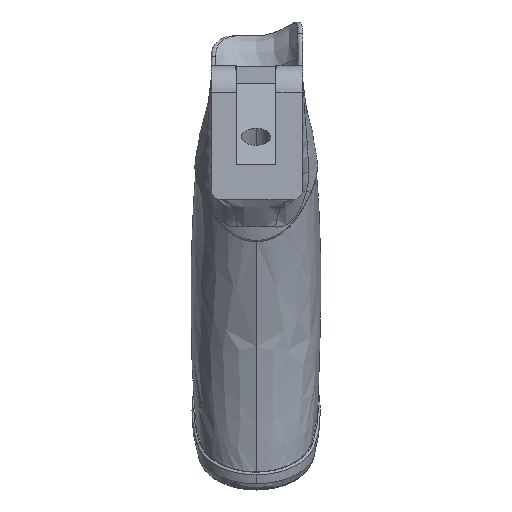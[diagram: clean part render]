
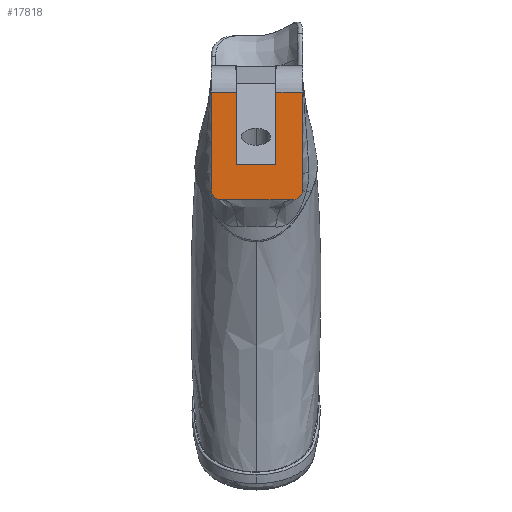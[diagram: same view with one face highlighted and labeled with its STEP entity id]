
A CAD part, top view. The second image highlights one B-rep face of the part: STEP entity #17818.
In plain terms, the highlighted planar face has unit normal (0, 0, 1).
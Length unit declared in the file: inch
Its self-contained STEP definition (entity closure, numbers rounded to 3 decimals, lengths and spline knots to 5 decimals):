
#292 = PLANE ( 'NONE',  #8919 ) ;
#348 = DIRECTION ( 'NONE',  ( 1., 0., 0. ) ) ;
#401 = CARTESIAN_POINT ( 'NONE',  ( -0.33, -1.2789, 0. ) ) ;
#866 = VERTEX_POINT ( 'NONE', #1141 ) ;
#1141 = CARTESIAN_POINT ( 'NONE',  ( 0.1875, -0.94, 0. ) ) ;
#1233 = CARTESIAN_POINT ( 'NONE',  ( 0.445, -1.1789, 0. ) ) ;
#1634 = VERTEX_POINT ( 'NONE', #8011 ) ;
#2180 = LINE ( 'NONE', #17868, #17293 ) ;
#2700 = CARTESIAN_POINT ( 'NONE',  ( -0.1875, -0.94, 0. ) ) ;
#2798 = CARTESIAN_POINT ( 'NONE',  ( 0.445, -0.25, 0. ) ) ;
#3036 = VERTEX_POINT ( 'NONE', #12469 ) ;
#3567 = EDGE_CURVE ( 'NONE', #1634, #18381, #17634, .T. ) ;
#3691 = EDGE_CURVE ( 'NONE', #8930, #7070, #12722, .T. ) ;
#3757 = ORIENTED_EDGE ( 'NONE', *, *, #21310, .T. ) ;
#4461 = LINE ( 'NONE', #8120, #19460 ) ;
#4905 = VECTOR ( 'NONE', #11008, 39.37008 ) ;
#4977 = CARTESIAN_POINT ( 'NONE',  ( 0.345, -1.2789, 0. ) ) ;
#5373 = EDGE_CURVE ( 'NONE', #12791, #10853, #4461, .T. ) ;
#5649 = CARTESIAN_POINT ( 'NONE',  ( 0.445, -1.2789, 0. ) ) ;
#5703 = DIRECTION ( 'NONE',  ( 1., 0., 0. ) ) ;
#5760 = CARTESIAN_POINT ( 'NONE',  ( -0.43, -1.2789, 0. ) ) ;
#5853 =( BOUNDED_CURVE ( )  B_SPLINE_CURVE ( 2, ( #7302, #14259, #401 ),
 .UNSPECIFIED., .F., .F. ) 
 B_SPLINE_CURVE_WITH_KNOTS ( ( 3, 3 ),
 ( 0., 0.00397 ),
 .UNSPECIFIED. ) 
 CURVE ( )  GEOMETRIC_REPRESENTATION_ITEM ( )  RATIONAL_B_SPLINE_CURVE ( ( 1., 0.707, 1. ) ) 
 REPRESENTATION_ITEM ( '' )  );
#5984 = VECTOR ( 'NONE', #14733, 39.37008 ) ;
#6343 = VECTOR ( 'NONE', #21409, 39.37008 ) ;
#7070 = VERTEX_POINT ( 'NONE', #1233 ) ;
#7084 = VECTOR ( 'NONE', #5703, 39.37008 ) ;
#7299 = FACE_OUTER_BOUND ( 'NONE', #9375, .T. ) ;
#7302 = CARTESIAN_POINT ( 'NONE',  ( -0.43, -1.1789, 0. ) ) ;
#7362 = CARTESIAN_POINT ( 'NONE',  ( 0.445, -1.1789, 0. ) ) ;
#7411 = LINE ( 'NONE', #21350, #7084 ) ;
#7652 = ORIENTED_EDGE ( 'NONE', *, *, #3567, .T. ) ;
#7694 = CARTESIAN_POINT ( 'NONE',  ( 0.345, -1.2789, 0. ) ) ;
#7800 = LINE ( 'NONE', #13050, #6343 ) ;
#7976 = ORIENTED_EDGE ( 'NONE', *, *, #8383, .T. ) ;
#8011 = CARTESIAN_POINT ( 'NONE',  ( -0.33, -1.2789, 0. ) ) ;
#8120 = CARTESIAN_POINT ( 'NONE',  ( -0.43, -0.25, 0. ) ) ;
#8383 = EDGE_CURVE ( 'NONE', #22419, #1634, #5853, .T. ) ;
#8904 = VECTOR ( 'NONE', #10793, 39.37008 ) ;
#8919 = AXIS2_PLACEMENT_3D ( 'NONE', #14146, #21018, #21465 ) ;
#8930 = VERTEX_POINT ( 'NONE', #2798 ) ;
#9195 = DIRECTION ( 'NONE',  ( 0., -1., 0. ) ) ;
#9375 = EDGE_LOOP ( 'NONE', ( #7652, #12896, #21637, #14820, #3757, #13836, #21369, #16314, #12779, #7976 ) ) ;
#10793 = DIRECTION ( 'NONE',  ( 0., -1., 0. ) ) ;
#10853 = VERTEX_POINT ( 'NONE', #13248 ) ;
#10969 = EDGE_CURVE ( 'NONE', #10853, #13007, #11195, .T. ) ;
#11008 = DIRECTION ( 'NONE',  ( 1., 0., 0. ) ) ;
#11073 = VECTOR ( 'NONE', #348, 39.37008 ) ;
#11195 = LINE ( 'NONE', #11308, #5984 ) ;
#11282 = EDGE_CURVE ( 'NONE', #12791, #22419, #7800, .T. ) ;
#11308 = CARTESIAN_POINT ( 'NONE',  ( -0.1875, 0., 0. ) ) ;
#11316 = EDGE_CURVE ( 'NONE', #18381, #7070, #16041, .T. ) ;
#12469 = CARTESIAN_POINT ( 'NONE',  ( 0.1875, -0.25, 0. ) ) ;
#12722 = LINE ( 'NONE', #17978, #8904 ) ;
#12723 = CARTESIAN_POINT ( 'NONE',  ( -0.1875, -0.94, 0. ) ) ;
#12779 = ORIENTED_EDGE ( 'NONE', *, *, #11282, .T. ) ;
#12791 = VERTEX_POINT ( 'NONE', #18049 ) ;
#12896 = ORIENTED_EDGE ( 'NONE', *, *, #11316, .T. ) ;
#13007 = VERTEX_POINT ( 'NONE', #2700 ) ;
#13050 = CARTESIAN_POINT ( 'NONE',  ( -0.43, -0.25, 0. ) ) ;
#13248 = CARTESIAN_POINT ( 'NONE',  ( -0.1875, -0.25, 0. ) ) ;
#13836 = ORIENTED_EDGE ( 'NONE', *, *, #21440, .F. ) ;
#14146 = CARTESIAN_POINT ( 'NONE',  ( -0.43, -0.25, 0. ) ) ;
#14259 = CARTESIAN_POINT ( 'NONE',  ( -0.43, -1.2789, 0. ) ) ;
#14430 = LINE ( 'NONE', #12723, #4905 ) ;
#14733 = DIRECTION ( 'NONE',  ( 0., -1., 0. ) ) ;
#14820 = ORIENTED_EDGE ( 'NONE', *, *, #18083, .F. ) ;
#15066 = DIRECTION ( 'NONE',  ( 1., 0., 0. ) ) ;
#16041 =( BOUNDED_CURVE ( )  B_SPLINE_CURVE ( 2, ( #7694, #5649, #7362 ),
 .UNSPECIFIED., .F., .F. ) 
 B_SPLINE_CURVE_WITH_KNOTS ( ( 3, 3 ),
 ( 0., 0.00397 ),
 .UNSPECIFIED. ) 
 CURVE ( )  GEOMETRIC_REPRESENTATION_ITEM ( )  RATIONAL_B_SPLINE_CURVE ( ( 1., 0.707, 1. ) ) 
 REPRESENTATION_ITEM ( '' )  );
#16314 = ORIENTED_EDGE ( 'NONE', *, *, #5373, .F. ) ;
#17293 = VECTOR ( 'NONE', #9195, 39.37008 ) ;
#17634 = LINE ( 'NONE', #5760, #11073 ) ;
#17818 = ADVANCED_FACE ( 'NONE', ( #7299 ), #292, .T. ) ;
#17868 = CARTESIAN_POINT ( 'NONE',  ( 0.1875, 0., 0. ) ) ;
#17978 = CARTESIAN_POINT ( 'NONE',  ( 0.445, -0.25, 0. ) ) ;
#18049 = CARTESIAN_POINT ( 'NONE',  ( -0.43, -0.25, 0. ) ) ;
#18083 = EDGE_CURVE ( 'NONE', #3036, #8930, #7411, .T. ) ;
#18381 = VERTEX_POINT ( 'NONE', #4977 ) ;
#19460 = VECTOR ( 'NONE', #15066, 39.37008 ) ;
#20493 = CARTESIAN_POINT ( 'NONE',  ( -0.43, -1.1789, 0. ) ) ;
#21018 = DIRECTION ( 'NONE',  ( 0., 0., 1. ) ) ;
#21310 = EDGE_CURVE ( 'NONE', #3036, #866, #2180, .T. ) ;
#21350 = CARTESIAN_POINT ( 'NONE',  ( -0.43, -0.25, 0. ) ) ;
#21369 = ORIENTED_EDGE ( 'NONE', *, *, #10969, .F. ) ;
#21409 = DIRECTION ( 'NONE',  ( 0., -1., 0. ) ) ;
#21440 = EDGE_CURVE ( 'NONE', #13007, #866, #14430, .T. ) ;
#21465 = DIRECTION ( 'NONE',  ( 0., -1., 0. ) ) ;
#21637 = ORIENTED_EDGE ( 'NONE', *, *, #3691, .F. ) ;
#22419 = VERTEX_POINT ( 'NONE', #20493 ) ;
